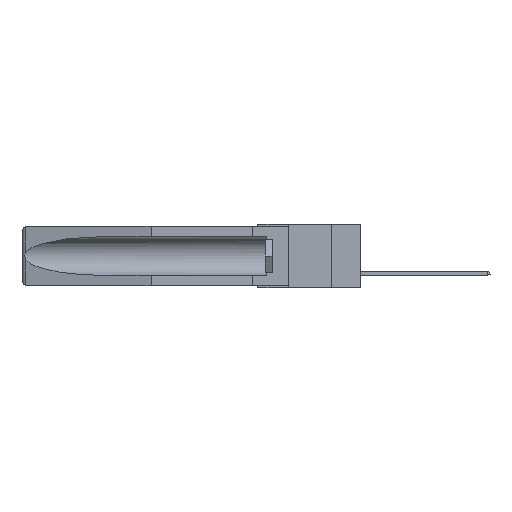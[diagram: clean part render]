
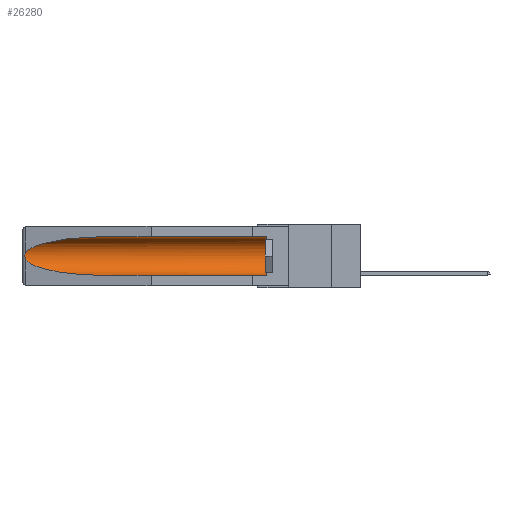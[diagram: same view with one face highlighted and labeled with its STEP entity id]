
A CAD part, left-side view. The second image highlights one B-rep face of the part: STEP entity #26280.
In plain terms, the highlighted cylindrical face has radius 2.857 mm (diameter 5.715 mm), a partial arc.
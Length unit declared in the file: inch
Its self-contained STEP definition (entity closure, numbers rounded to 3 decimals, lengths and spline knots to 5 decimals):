
#600 = ORIENTED_EDGE ( 'NONE', *, *, #15497, .T. ) ;
#778 = VERTEX_POINT ( 'NONE', #22927 ) ;
#1704 = FACE_OUTER_BOUND ( 'NONE', #10052, .T. ) ;
#1874 = EDGE_CURVE ( 'NONE', #778, #19591, #30149, .T. ) ;
#2251 = VERTEX_POINT ( 'NONE', #10027 ) ;
#3697 = ORIENTED_EDGE ( 'NONE', *, *, #15192, .T. ) ;
#3780 = CARTESIAN_POINT ( 'NONE',  ( 0.26537, 1.52718, -0.19328 ) ) ;
#3998 = CARTESIAN_POINT ( 'NONE',  ( 0.2675, 1.53308, -0.17534 ) ) ;
#4867 = ORIENTED_EDGE ( 'NONE', *, *, #1874, .T. ) ;
#4911 = CARTESIAN_POINT ( 'NONE',  ( 0.155, -0.30754, -0.284 ) ) ;
#5033 = CYLINDRICAL_SURFACE ( 'NONE', #6076, 0.1125 ) ;
#5430 = CARTESIAN_POINT ( 'NONE',  ( 0.155, -0.30754, -0.1715 ) ) ;
#5438 = ORIENTED_EDGE ( 'NONE', *, *, #12867, .T. ) ;
#6076 = AXIS2_PLACEMENT_3D ( 'NONE', #5430, #14670, #29156 ) ;
#8274 = CARTESIAN_POINT ( 'NONE',  ( 0.26537, 1.52718, -0.14972 ) ) ;
#8316 = CARTESIAN_POINT ( 'NONE',  ( 0.26537, 1.52718, -0.19328 ) ) ;
#8485 = CARTESIAN_POINT ( 'NONE',  ( 0.26655, 1.53094, -0.18657 ) ) ;
#8591 = VERTEX_POINT ( 'NONE', #8316 ) ;
#8966 = VECTOR ( 'NONE', #23881, 39.37008 ) ;
#10027 = CARTESIAN_POINT ( 'NONE',  ( 0.155, 0.126, -0.284 ) ) ;
#10052 = EDGE_LOOP ( 'NONE', ( #4867, #3697, #5438, #29258, #13625, #600 ) ) ;
#10169 = CARTESIAN_POINT ( 'NONE',  ( 0.26597, 1.52961, -0.15275 ) ) ;
#11043 = CARTESIAN_POINT ( 'NONE',  ( 0.26537, 1.52718, -0.14972 ) ) ;
#12419 = CARTESIAN_POINT ( 'NONE',  ( 0.26537, 1.52718, -0.14972 ) ) ;
#12533 = CARTESIAN_POINT ( 'NONE',  ( 0.2675, 1.53308, -0.16763 ) ) ;
#12867 = EDGE_CURVE ( 'NONE', #8591, #24534, #26888, .T. ) ;
#13117 = CARTESIAN_POINT ( 'NONE',  ( 0.2673, 1.53269, -0.17917 ) ) ;
#13625 = ORIENTED_EDGE ( 'NONE', *, *, #13976, .T. ) ;
#13746 = CIRCLE ( 'NONE', #29100, 0.1125 ) ;
#13976 = EDGE_CURVE ( 'NONE', #2251, #27206, #13746, .T. ) ;
#14121 = CARTESIAN_POINT ( 'NONE',  ( 0.26537, 1.52718, -0.19328 ) ) ;
#14670 = DIRECTION ( 'NONE',  ( 0., 1., 0. ) ) ;
#14904 = CARTESIAN_POINT ( 'NONE',  ( 0.155, 1.07973, -0.284 ) ) ;
#14919 = CARTESIAN_POINT ( 'NONE',  ( 0.26654, 1.53092, -0.15636 ) ) ;
#15192 = EDGE_CURVE ( 'NONE', #19591, #8591, #24055, .T. ) ;
#15497 = EDGE_CURVE ( 'NONE', #27206, #778, #18776, .T. ) ;
#15865 = CARTESIAN_POINT ( 'NONE',  ( 0.155, 1.07973, -0.284 ) ) ;
#16393 = CARTESIAN_POINT ( 'NONE',  ( 0.155, 0.126, -0.1715 ) ) ;
#18776 = LINE ( 'NONE', #20154, #25815 ) ;
#19096 = CARTESIAN_POINT ( 'NONE',  ( 0.25451, 1.48313, -0.24835 ) ) ;
#19591 = VERTEX_POINT ( 'NONE', #11043 ) ;
#19822 = EDGE_CURVE ( 'NONE', #2251, #24534, #22294, .T. ) ;
#20072 = CARTESIAN_POINT ( 'NONE',  ( 0.155, 1.07973, -0.059 ) ) ;
#20154 = CARTESIAN_POINT ( 'NONE',  ( 0.155, -0.30754, -0.059 ) ) ;
#20576 = CARTESIAN_POINT ( 'NONE',  ( 0.26597, 1.5296, -0.19026 ) ) ;
#22294 = LINE ( 'NONE', #4911, #8966 ) ;
#22469 = CARTESIAN_POINT ( 'NONE',  ( 0.21114, 1.30732, -0.059 ) ) ;
#22927 = CARTESIAN_POINT ( 'NONE',  ( 0.155, 1.07973, -0.059 ) ) ;
#23137 = CARTESIAN_POINT ( 'NONE',  ( 0.21114, 1.30732, -0.284 ) ) ;
#23535 = CARTESIAN_POINT ( 'NONE',  ( 0.155, 0.126, -0.059 ) ) ;
#23881 = DIRECTION ( 'NONE',  ( 0., 1., 0. ) ) ;
#24055 = B_SPLINE_CURVE_WITH_KNOTS ( 'NONE', 3,
 ( #12419, #10169, #14919, #26702, #12533, #3998, #13117, #8485, #20576, #3780 ),
 .UNSPECIFIED., .F., .F.,
 ( 4, 2, 2, 2, 4 ),
 ( 0., 0.00029, 0.00058, 0.00087, 0.00117 ),
 .UNSPECIFIED. ) ;
#24534 = VERTEX_POINT ( 'NONE', #14904 ) ;
#24830 = CARTESIAN_POINT ( 'NONE',  ( 0.25451, 1.48313, -0.09465 ) ) ;
#25815 = VECTOR ( 'NONE', #27390, 39.37008 ) ;
#25934 = DIRECTION ( 'NONE',  ( 0., -1., 0. ) ) ;
#26280 = ADVANCED_FACE ( 'NONE', ( #1704 ), #5033, .F. ) ;
#26702 = CARTESIAN_POINT ( 'NONE',  ( 0.2673, 1.5327, -0.16383 ) ) ;
#26888 =( BOUNDED_CURVE ( )  B_SPLINE_CURVE ( 3, ( #14121, #19096, #23137, #15865 ),
 .UNSPECIFIED., .F., .F. ) 
 B_SPLINE_CURVE_WITH_KNOTS ( ( 4, 4 ),
 ( 0.1948, 1.5708 ),
 .UNSPECIFIED. ) 
 CURVE ( )  GEOMETRIC_REPRESENTATION_ITEM ( )  RATIONAL_B_SPLINE_CURVE ( ( 1., 0.848, 0.848, 1. ) ) 
 REPRESENTATION_ITEM ( '' )  );
#27206 = VERTEX_POINT ( 'NONE', #23535 ) ;
#27390 = DIRECTION ( 'NONE',  ( 0., 1., 0. ) ) ;
#28323 = DIRECTION ( 'NONE',  ( 0., 0., 1. ) ) ;
#29100 = AXIS2_PLACEMENT_3D ( 'NONE', #16393, #25934, #28323 ) ;
#29156 = DIRECTION ( 'NONE',  ( 0., 0., 1. ) ) ;
#29258 = ORIENTED_EDGE ( 'NONE', *, *, #19822, .F. ) ;
#30149 =( BOUNDED_CURVE ( )  B_SPLINE_CURVE ( 3, ( #20072, #22469, #24830, #8274 ),
 .UNSPECIFIED., .F., .F. ) 
 B_SPLINE_CURVE_WITH_KNOTS ( ( 4, 4 ),
 ( 4.71239, 6.08839 ),
 .UNSPECIFIED. ) 
 CURVE ( )  GEOMETRIC_REPRESENTATION_ITEM ( )  RATIONAL_B_SPLINE_CURVE ( ( 1., 0.848, 0.848, 1. ) ) 
 REPRESENTATION_ITEM ( '' )  );
